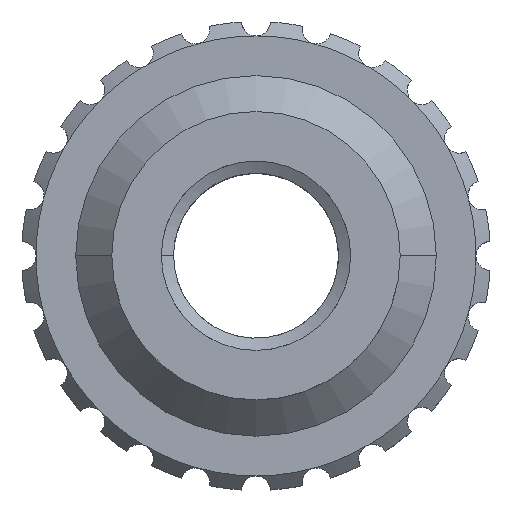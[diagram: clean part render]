
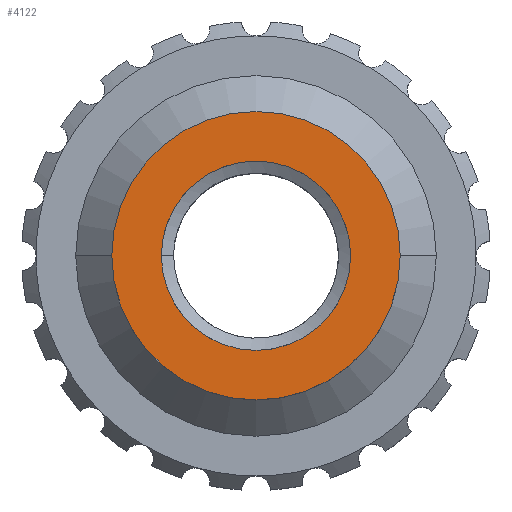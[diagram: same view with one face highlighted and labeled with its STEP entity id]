
A CAD part, top view. The second image highlights one B-rep face of the part: STEP entity #4122.
In plain terms, the highlighted planar face has unit normal (0, 0, 1).
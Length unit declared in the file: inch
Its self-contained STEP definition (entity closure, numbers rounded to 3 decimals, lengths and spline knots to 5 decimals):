
#66 = EDGE_LOOP ( 'NONE', ( #4797, #3284 ) ) ;
#555 = CARTESIAN_POINT ( 'NONE',  ( 0.1167, -0.38462, -1.25087 ) ) ;
#592 = DIRECTION ( 'NONE',  ( 0., 0., 1. ) ) ;
#861 = ORIENTED_EDGE ( 'NONE', *, *, #1606, .T. ) ;
#889 = FACE_OUTER_BOUND ( 'NONE', #4651, .T. ) ;
#908 = DIRECTION ( 'NONE',  ( 1., 0., 0. ) ) ;
#966 = CIRCLE ( 'NONE', #1106, 0.13125 ) ;
#1003 = CARTESIAN_POINT ( 'NONE',  ( 0.44795, -0.38462, -1.25087 ) ) ;
#1066 = AXIS2_PLACEMENT_3D ( 'NONE', #2098, #5452, #1222 ) ;
#1106 = AXIS2_PLACEMENT_3D ( 'NONE', #4163, #1359, #4233 ) ;
#1222 = DIRECTION ( 'NONE',  ( 1., 0., 0. ) ) ;
#1359 = DIRECTION ( 'NONE',  ( 0., 0., 1. ) ) ;
#1546 = CIRCLE ( 'NONE', #3360, 0.13125 ) ;
#1578 = PLANE ( 'NONE',  #3661 ) ;
#1606 = EDGE_CURVE ( 'NONE', #5123, #5849, #1843, .T. ) ;
#1843 = CIRCLE ( 'NONE', #1066, 0.2 ) ;
#1916 = CARTESIAN_POINT ( 'NONE',  ( 0.24795, -0.38462, -1.25087 ) ) ;
#2098 = CARTESIAN_POINT ( 'NONE',  ( 0.24795, -0.38462, -1.25087 ) ) ;
#2384 = DIRECTION ( 'NONE',  ( 1., 0., 0. ) ) ;
#2806 = CIRCLE ( 'NONE', #3772, 0.2 ) ;
#3188 = CARTESIAN_POINT ( 'NONE',  ( 0.24795, -0.38462, -1.25087 ) ) ;
#3194 = CARTESIAN_POINT ( 'NONE',  ( 0.04795, -0.38462, -1.25087 ) ) ;
#3284 = ORIENTED_EDGE ( 'NONE', *, *, #5259, .F. ) ;
#3360 = AXIS2_PLACEMENT_3D ( 'NONE', #3188, #5530, #908 ) ;
#3626 = EDGE_CURVE ( 'NONE', #4802, #4947, #966, .T. ) ;
#3661 = AXIS2_PLACEMENT_3D ( 'NONE', #4421, #592, #5842 ) ;
#3772 = AXIS2_PLACEMENT_3D ( 'NONE', #1916, #5269, #2384 ) ;
#3827 = EDGE_CURVE ( 'NONE', #5849, #5123, #2806, .T. ) ;
#4122 = ADVANCED_FACE ( 'NONE', ( #4326, #889 ), #1578, .T. ) ;
#4163 = CARTESIAN_POINT ( 'NONE',  ( 0.24795, -0.38462, -1.25087 ) ) ;
#4233 = DIRECTION ( 'NONE',  ( 1., 0., 0. ) ) ;
#4326 = FACE_BOUND ( 'NONE', #66, .T. ) ;
#4421 = CARTESIAN_POINT ( 'NONE',  ( 0.24795, -0.38462, -1.25087 ) ) ;
#4651 = EDGE_LOOP ( 'NONE', ( #5620, #861 ) ) ;
#4797 = ORIENTED_EDGE ( 'NONE', *, *, #3626, .F. ) ;
#4802 = VERTEX_POINT ( 'NONE', #555 ) ;
#4947 = VERTEX_POINT ( 'NONE', #5200 ) ;
#5123 = VERTEX_POINT ( 'NONE', #1003 ) ;
#5200 = CARTESIAN_POINT ( 'NONE',  ( 0.3792, -0.38462, -1.25087 ) ) ;
#5259 = EDGE_CURVE ( 'NONE', #4947, #4802, #1546, .T. ) ;
#5269 = DIRECTION ( 'NONE',  ( 0., 0., 1. ) ) ;
#5452 = DIRECTION ( 'NONE',  ( 0., 0., 1. ) ) ;
#5530 = DIRECTION ( 'NONE',  ( 0., 0., 1. ) ) ;
#5620 = ORIENTED_EDGE ( 'NONE', *, *, #3827, .T. ) ;
#5842 = DIRECTION ( 'NONE',  ( 1., 0., 0. ) ) ;
#5849 = VERTEX_POINT ( 'NONE', #3194 ) ;
